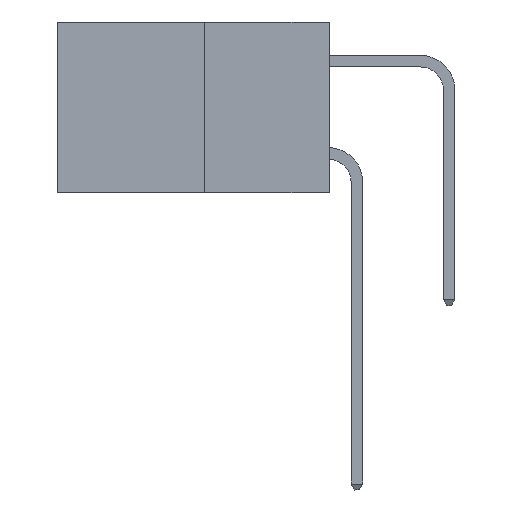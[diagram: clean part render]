
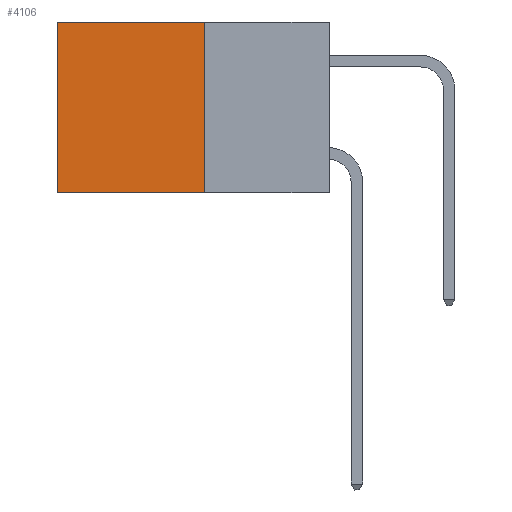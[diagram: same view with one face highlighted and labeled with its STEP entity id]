
A CAD part, left-side view. The second image highlights one B-rep face of the part: STEP entity #4106.
In plain terms, the highlighted planar face has unit normal (-1, 0, 0).
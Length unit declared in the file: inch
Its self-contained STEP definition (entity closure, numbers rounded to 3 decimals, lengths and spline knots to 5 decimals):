
#115 = DIRECTION ( 'NONE',  ( 0., 0., -1. ) ) ;
#503 = DIRECTION ( 'NONE',  ( 0., 0., -1. ) ) ;
#553 = CARTESIAN_POINT ( 'NONE',  ( 0.277, 0.59, 0. ) ) ;
#791 = CARTESIAN_POINT ( 'NONE',  ( 0.277, 0.27, -0.37 ) ) ;
#1375 = EDGE_CURVE ( 'NONE', #2889, #1478, #8041, .T. ) ;
#1421 = CARTESIAN_POINT ( 'NONE',  ( 0.277, 0.27, -0.37 ) ) ;
#1478 = VERTEX_POINT ( 'NONE', #2696 ) ;
#1908 = LINE ( 'NONE', #1421, #3678 ) ;
#1984 = CARTESIAN_POINT ( 'NONE',  ( 0.277, 0.27, -0.37 ) ) ;
#2498 = DIRECTION ( 'NONE',  ( 0., 1., 0. ) ) ;
#2696 = CARTESIAN_POINT ( 'NONE',  ( 0.277, 0.59, -0.37 ) ) ;
#2889 = VERTEX_POINT ( 'NONE', #553 ) ;
#3298 = VECTOR ( 'NONE', #6397, 39.37008 ) ;
#3650 = VERTEX_POINT ( 'NONE', #791 ) ;
#3678 = VECTOR ( 'NONE', #2498, 39.37008 ) ;
#4053 = PLANE ( 'NONE',  #8841 ) ;
#4106 = ADVANCED_FACE ( 'NONE', ( #4335 ), #4053, .F. ) ;
#4162 = VECTOR ( 'NONE', #503, 39.37008 ) ;
#4335 = FACE_OUTER_BOUND ( 'NONE', #9340, .T. ) ;
#4572 = DIRECTION ( 'NONE',  ( 1., 0., 0. ) ) ;
#5243 = EDGE_CURVE ( 'NONE', #3650, #1478, #1908, .T. ) ;
#5301 = ORIENTED_EDGE ( 'NONE', *, *, #1375, .T. ) ;
#6116 = CARTESIAN_POINT ( 'NONE',  ( 0.277, 0.27, 0. ) ) ;
#6397 = DIRECTION ( 'NONE',  ( 0., 1., 0. ) ) ;
#6671 = EDGE_CURVE ( 'NONE', #9164, #2889, #6879, .T. ) ;
#6856 = VECTOR ( 'NONE', #115, 39.37008 ) ;
#6879 = LINE ( 'NONE', #6116, #3298 ) ;
#7138 = ORIENTED_EDGE ( 'NONE', *, *, #6671, .T. ) ;
#7488 = DIRECTION ( 'NONE',  ( 0., 0., -1. ) ) ;
#7552 = EDGE_CURVE ( 'NONE', #9164, #3650, #8775, .T. ) ;
#7719 = CARTESIAN_POINT ( 'NONE',  ( 0.277, 0.59, -0.37 ) ) ;
#8041 = LINE ( 'NONE', #7719, #4162 ) ;
#8276 = CARTESIAN_POINT ( 'NONE',  ( 0.277, 0.27, -0.37 ) ) ;
#8518 = CARTESIAN_POINT ( 'NONE',  ( 0.277, 0.27, 0. ) ) ;
#8633 = ORIENTED_EDGE ( 'NONE', *, *, #5243, .F. ) ;
#8775 = LINE ( 'NONE', #8276, #6856 ) ;
#8841 = AXIS2_PLACEMENT_3D ( 'NONE', #1984, #4572, #7488 ) ;
#9164 = VERTEX_POINT ( 'NONE', #8518 ) ;
#9340 = EDGE_LOOP ( 'NONE', ( #5301, #8633, #9355, #7138 ) ) ;
#9355 = ORIENTED_EDGE ( 'NONE', *, *, #7552, .F. ) ;
